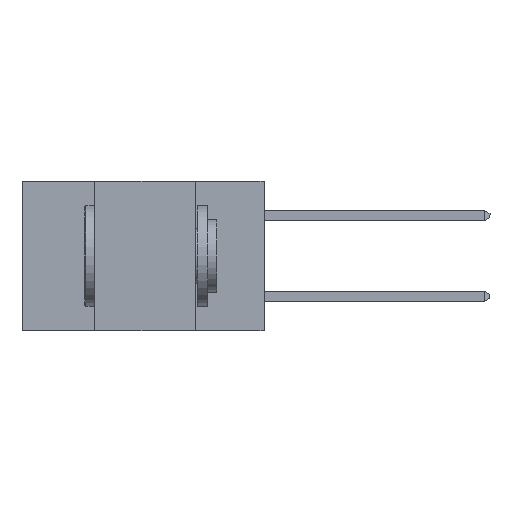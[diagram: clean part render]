
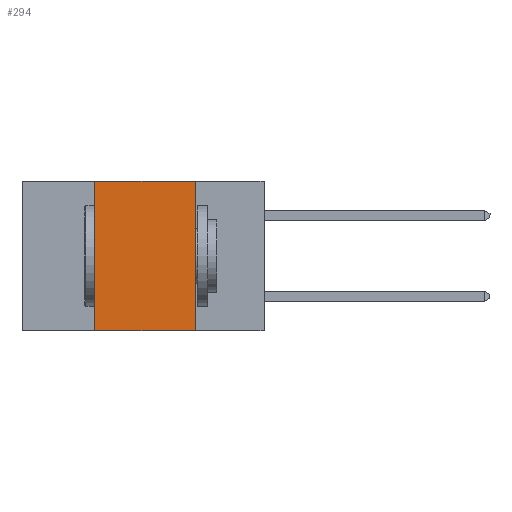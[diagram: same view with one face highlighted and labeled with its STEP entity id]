
A CAD part, left-side view. The second image highlights one B-rep face of the part: STEP entity #294.
In plain terms, the highlighted planar face has unit normal (-1, 0, 0).
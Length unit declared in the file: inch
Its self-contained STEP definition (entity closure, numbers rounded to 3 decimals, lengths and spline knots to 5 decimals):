
#294 = ADVANCED_FACE ( 'NONE', ( #27696 ), #11258, .F. ) ;
#770 = VERTEX_POINT ( 'NONE', #1612 ) ;
#1612 = CARTESIAN_POINT ( 'NONE',  ( 0., 0.42, -0.37 ) ) ;
#2144 = VECTOR ( 'NONE', #9148, 39.37008 ) ;
#3245 = LINE ( 'NONE', #12884, #4720 ) ;
#3950 = CARTESIAN_POINT ( 'NONE',  ( 0., 0.42, 0. ) ) ;
#4354 = EDGE_CURVE ( 'NONE', #7421, #28711, #26133, .T. ) ;
#4720 = VECTOR ( 'NONE', #15188, 39.37008 ) ;
#5290 = ORIENTED_EDGE ( 'NONE', *, *, #8618, .F. ) ;
#6731 = ORIENTED_EDGE ( 'NONE', *, *, #8890, .T. ) ;
#7421 = VERTEX_POINT ( 'NONE', #12845 ) ;
#8063 = VECTOR ( 'NONE', #16629, 39.37008 ) ;
#8618 = EDGE_CURVE ( 'NONE', #770, #17560, #3245, .T. ) ;
#8890 = EDGE_CURVE ( 'NONE', #770, #28711, #20439, .T. ) ;
#9148 = DIRECTION ( 'NONE',  ( 0., -1., 0. ) ) ;
#10463 = DIRECTION ( 'NONE',  ( 1., 0., 0. ) ) ;
#10525 = DIRECTION ( 'NONE',  ( 0., 0., -1. ) ) ;
#11119 = EDGE_CURVE ( 'NONE', #17560, #7421, #24804, .T. ) ;
#11258 = PLANE ( 'NONE',  #24563 ) ;
#12845 = CARTESIAN_POINT ( 'NONE',  ( 0., 0.17, 0. ) ) ;
#12884 = CARTESIAN_POINT ( 'NONE',  ( 0., 0.42, 0. ) ) ;
#15188 = DIRECTION ( 'NONE',  ( 0., 0., 1. ) ) ;
#15315 = ORIENTED_EDGE ( 'NONE', *, *, #4354, .F. ) ;
#15463 = EDGE_LOOP ( 'NONE', ( #15315, #16037, #5290, #6731 ) ) ;
#16037 = ORIENTED_EDGE ( 'NONE', *, *, #11119, .F. ) ;
#16629 = DIRECTION ( 'NONE',  ( 0., -1., 0. ) ) ;
#17560 = VERTEX_POINT ( 'NONE', #3950 ) ;
#18201 = CARTESIAN_POINT ( 'NONE',  ( 0., 0.17, -0.37 ) ) ;
#20439 = LINE ( 'NONE', #27225, #2144 ) ;
#20661 = DIRECTION ( 'NONE',  ( 0., 0., -1. ) ) ;
#20926 = CARTESIAN_POINT ( 'NONE',  ( 0., 0.17, 0. ) ) ;
#21271 = CARTESIAN_POINT ( 'NONE',  ( 0., 0.6, 0. ) ) ;
#21562 = CARTESIAN_POINT ( 'NONE',  ( 0., 0.6, 0. ) ) ;
#24563 = AXIS2_PLACEMENT_3D ( 'NONE', #21562, #10463, #10525 ) ;
#24718 = VECTOR ( 'NONE', #20661, 39.37008 ) ;
#24804 = LINE ( 'NONE', #21271, #8063 ) ;
#26133 = LINE ( 'NONE', #20926, #24718 ) ;
#27225 = CARTESIAN_POINT ( 'NONE',  ( 0., 0.6, -0.37 ) ) ;
#27696 = FACE_OUTER_BOUND ( 'NONE', #15463, .T. ) ;
#28711 = VERTEX_POINT ( 'NONE', #18201 ) ;
